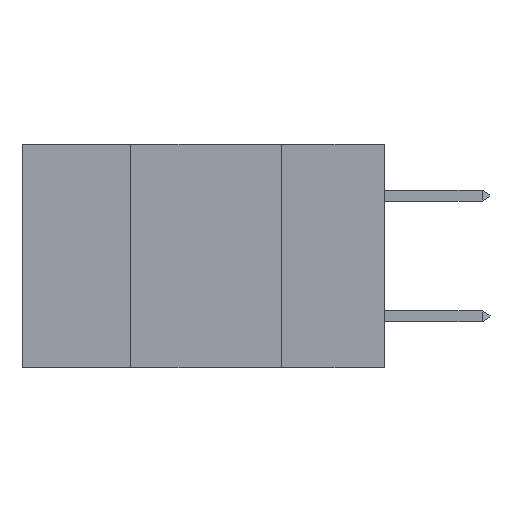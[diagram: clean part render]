
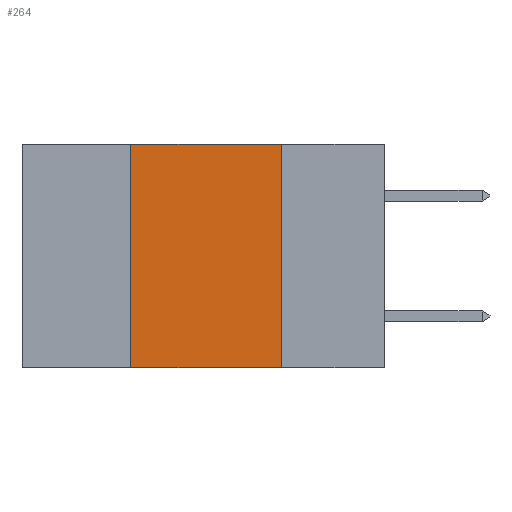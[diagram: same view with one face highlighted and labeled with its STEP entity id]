
A CAD part, left-side view. The second image highlights one B-rep face of the part: STEP entity #264.
In plain terms, the highlighted planar face has unit normal (-1, 0, 0).
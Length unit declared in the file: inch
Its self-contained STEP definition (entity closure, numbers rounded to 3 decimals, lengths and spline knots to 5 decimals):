
#264 = ADVANCED_FACE ( 'NONE', ( #5649 ), #470, .F. ) ;
#322 = VERTEX_POINT ( 'NONE', #10090 ) ;
#323 = CARTESIAN_POINT ( 'NONE',  ( 0., 0.6, -0.37 ) ) ;
#470 = PLANE ( 'NONE',  #7483 ) ;
#472 = DIRECTION ( 'NONE',  ( 0., 0., -1. ) ) ;
#591 = ORIENTED_EDGE ( 'NONE', *, *, #2439, .T. ) ;
#1011 = VERTEX_POINT ( 'NONE', #9868 ) ;
#1243 = LINE ( 'NONE', #4841, #3952 ) ;
#1404 = CARTESIAN_POINT ( 'NONE',  ( 0., 0.17, 0. ) ) ;
#2014 = DIRECTION ( 'NONE',  ( 0., -1., 0. ) ) ;
#2103 = LINE ( 'NONE', #9219, #6903 ) ;
#2439 = EDGE_CURVE ( 'NONE', #322, #6417, #3814, .T. ) ;
#2840 = VECTOR ( 'NONE', #2014, 39.37008 ) ;
#3814 = LINE ( 'NONE', #323, #2840 ) ;
#3824 = CARTESIAN_POINT ( 'NONE',  ( 0., 0.17, 0. ) ) ;
#3832 = ORIENTED_EDGE ( 'NONE', *, *, #7194, .F. ) ;
#3952 = VECTOR ( 'NONE', #3962, 39.37008 ) ;
#3962 = DIRECTION ( 'NONE',  ( 0., 0., 1. ) ) ;
#4107 = CARTESIAN_POINT ( 'NONE',  ( 0., 0.17, -0.37 ) ) ;
#4778 = DIRECTION ( 'NONE',  ( 0., -1., 0. ) ) ;
#4830 = CARTESIAN_POINT ( 'NONE',  ( 0., 0.6, 0. ) ) ;
#4834 = ORIENTED_EDGE ( 'NONE', *, *, #9366, .F. ) ;
#4841 = CARTESIAN_POINT ( 'NONE',  ( 0., 0.42, 0. ) ) ;
#5586 = DIRECTION ( 'NONE',  ( 1., 0., 0. ) ) ;
#5649 = FACE_OUTER_BOUND ( 'NONE', #8410, .T. ) ;
#5911 = EDGE_CURVE ( 'NONE', #11521, #6417, #11091, .T. ) ;
#6417 = VERTEX_POINT ( 'NONE', #4107 ) ;
#6903 = VECTOR ( 'NONE', #4778, 39.37008 ) ;
#7194 = EDGE_CURVE ( 'NONE', #1011, #11521, #2103, .T. ) ;
#7483 = AXIS2_PLACEMENT_3D ( 'NONE', #4830, #5586, #7584 ) ;
#7584 = DIRECTION ( 'NONE',  ( 0., 0., -1. ) ) ;
#8410 = EDGE_LOOP ( 'NONE', ( #8546, #3832, #4834, #591 ) ) ;
#8546 = ORIENTED_EDGE ( 'NONE', *, *, #5911, .F. ) ;
#9219 = CARTESIAN_POINT ( 'NONE',  ( 0., 0.6, 0. ) ) ;
#9366 = EDGE_CURVE ( 'NONE', #322, #1011, #1243, .T. ) ;
#9626 = VECTOR ( 'NONE', #472, 39.37008 ) ;
#9868 = CARTESIAN_POINT ( 'NONE',  ( 0., 0.42, 0. ) ) ;
#10090 = CARTESIAN_POINT ( 'NONE',  ( 0., 0.42, -0.37 ) ) ;
#11091 = LINE ( 'NONE', #1404, #9626 ) ;
#11521 = VERTEX_POINT ( 'NONE', #3824 ) ;
